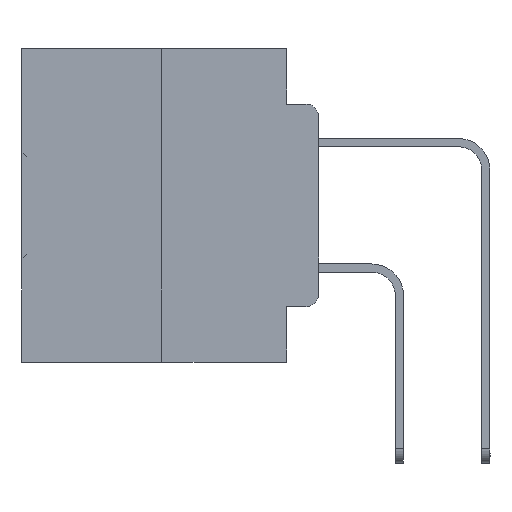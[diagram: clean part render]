
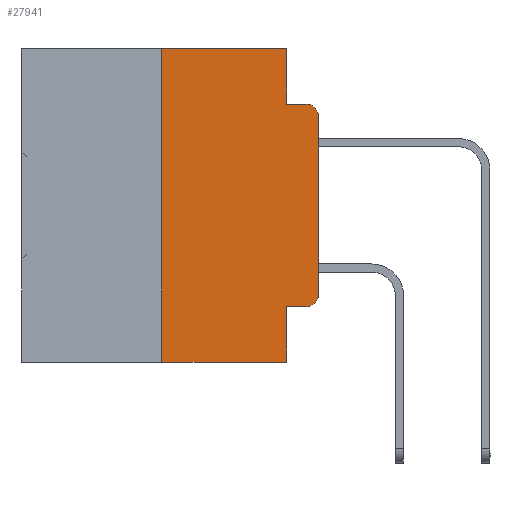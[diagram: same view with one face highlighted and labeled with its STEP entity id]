
A CAD part, left-side view. The second image highlights one B-rep face of the part: STEP entity #27941.
In plain terms, the highlighted planar face has unit normal (-1, 0, 0).
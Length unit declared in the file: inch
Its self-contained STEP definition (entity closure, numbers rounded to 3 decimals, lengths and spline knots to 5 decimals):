
#73 = CARTESIAN_POINT ( 'NONE',  ( 0., 0.051, 0. ) ) ;
#730 = ORIENTED_EDGE ( 'NONE', *, *, #11792, .T. ) ;
#1416 = CARTESIAN_POINT ( 'NONE',  ( 0., 0., -0.3915 ) ) ;
#2061 = DIRECTION ( 'NONE',  ( 0., -1., 0. ) ) ;
#2429 = VERTEX_POINT ( 'NONE', #34743 ) ;
#3399 = DIRECTION ( 'NONE',  ( 0., 0., 1. ) ) ;
#3607 = VECTOR ( 'NONE', #5566, 39.37008 ) ;
#4723 = FACE_OUTER_BOUND ( 'NONE', #28030, .T. ) ;
#5356 = ORIENTED_EDGE ( 'NONE', *, *, #24350, .F. ) ;
#5566 = DIRECTION ( 'NONE',  ( 0., -1., 0. ) ) ;
#7035 = ORIENTED_EDGE ( 'NONE', *, *, #22281, .T. ) ;
#7354 = ORIENTED_EDGE ( 'NONE', *, *, #14879, .F. ) ;
#7501 = LINE ( 'NONE', #73, #13988 ) ;
#7784 = VERTEX_POINT ( 'NONE', #1416 ) ;
#8069 = ORIENTED_EDGE ( 'NONE', *, *, #12528, .F. ) ;
#8354 = AXIS2_PLACEMENT_3D ( 'NONE', #11771, #9117, #33645 ) ;
#8865 = CARTESIAN_POINT ( 'NONE',  ( 0., 0.051, 0. ) ) ;
#8930 = LINE ( 'NONE', #35645, #33581 ) ;
#9117 = DIRECTION ( 'NONE',  ( -1., 0., 0. ) ) ;
#9199 = PLANE ( 'NONE',  #20997 ) ;
#9669 = CARTESIAN_POINT ( 'NONE',  ( 0., 0.25, -0.5 ) ) ;
#10560 = DIRECTION ( 'NONE',  ( 0., 0., -1. ) ) ;
#10842 = CARTESIAN_POINT ( 'NONE',  ( 0., 0.051, -0.4115 ) ) ;
#10954 = DIRECTION ( 'NONE',  ( 0., -1., 0. ) ) ;
#11186 = CARTESIAN_POINT ( 'NONE',  ( 0., 0.473, 0. ) ) ;
#11771 = CARTESIAN_POINT ( 'NONE',  ( 0., 0.02, -0.3915 ) ) ;
#11792 = EDGE_CURVE ( 'NONE', #2429, #7784, #31739, .T. ) ;
#11823 = LINE ( 'NONE', #16718, #3607 ) ;
#12345 = CARTESIAN_POINT ( 'NONE',  ( 0., 0.473, 0. ) ) ;
#12483 = ORIENTED_EDGE ( 'NONE', *, *, #35560, .T. ) ;
#12528 = EDGE_CURVE ( 'NONE', #12726, #15545, #35096, .T. ) ;
#12705 = CIRCLE ( 'NONE', #17532, 0.02 ) ;
#12726 = VERTEX_POINT ( 'NONE', #9669 ) ;
#13062 = VECTOR ( 'NONE', #3399, 39.37008 ) ;
#13065 = VERTEX_POINT ( 'NONE', #8865 ) ;
#13231 = DIRECTION ( 'NONE',  ( -1., 0., 0. ) ) ;
#13613 = CARTESIAN_POINT ( 'NONE',  ( 0., 0.051, -0.4115 ) ) ;
#13663 = CARTESIAN_POINT ( 'NONE',  ( 0., 0.051, -0.0885 ) ) ;
#13988 = VECTOR ( 'NONE', #19879, 39.37008 ) ;
#14879 = EDGE_CURVE ( 'NONE', #13065, #26936, #8930, .T. ) ;
#15179 = VECTOR ( 'NONE', #2061, 39.37008 ) ;
#15545 = VERTEX_POINT ( 'NONE', #25599 ) ;
#15902 = CARTESIAN_POINT ( 'NONE',  ( 0., 0.02, -0.1085 ) ) ;
#16213 = EDGE_CURVE ( 'NONE', #23597, #16334, #12705, .T. ) ;
#16334 = VERTEX_POINT ( 'NONE', #22217 ) ;
#16426 = EDGE_CURVE ( 'NONE', #21245, #32821, #7501, .T. ) ;
#16718 = CARTESIAN_POINT ( 'NONE',  ( 0., 0.473, -0.5 ) ) ;
#17532 = AXIS2_PLACEMENT_3D ( 'NONE', #15902, #13231, #10560 ) ;
#19879 = DIRECTION ( 'NONE',  ( 0., 0., -1. ) ) ;
#20142 = LINE ( 'NONE', #11186, #22800 ) ;
#20997 = AXIS2_PLACEMENT_3D ( 'NONE', #12345, #34086, #23163 ) ;
#21245 = VERTEX_POINT ( 'NONE', #10842 ) ;
#22035 = EDGE_CURVE ( 'NONE', #7784, #23597, #31540, .T. ) ;
#22217 = CARTESIAN_POINT ( 'NONE',  ( 0., 0.02, -0.0885 ) ) ;
#22281 = EDGE_CURVE ( 'NONE', #21245, #2429, #25498, .T. ) ;
#22606 = CARTESIAN_POINT ( 'NONE',  ( 0., 0.051, -0.5 ) ) ;
#22800 = VECTOR ( 'NONE', #10954, 39.37008 ) ;
#22900 = VECTOR ( 'NONE', #30199, 39.37008 ) ;
#23163 = DIRECTION ( 'NONE',  ( 0., 0., -1. ) ) ;
#23359 = CARTESIAN_POINT ( 'NONE',  ( 0., 0., 0. ) ) ;
#23594 = DIRECTION ( 'NONE',  ( 0., 0., 1. ) ) ;
#23597 = VERTEX_POINT ( 'NONE', #35299 ) ;
#24350 = EDGE_CURVE ( 'NONE', #15545, #13065, #20142, .T. ) ;
#24724 = DIRECTION ( 'NONE',  ( 0., 0., -1. ) ) ;
#25498 = LINE ( 'NONE', #13613, #22900 ) ;
#25534 = VECTOR ( 'NONE', #23594, 39.37008 ) ;
#25599 = CARTESIAN_POINT ( 'NONE',  ( 0., 0.25, 0. ) ) ;
#26299 = CARTESIAN_POINT ( 'NONE',  ( 0., 0.051, -0.0885 ) ) ;
#26606 = ORIENTED_EDGE ( 'NONE', *, *, #22035, .T. ) ;
#26936 = VERTEX_POINT ( 'NONE', #26299 ) ;
#27941 = ADVANCED_FACE ( 'NONE', ( #4723 ), #9199, .F. ) ;
#28030 = EDGE_LOOP ( 'NONE', ( #26606, #29717, #30797, #7354, #5356, #8069, #12483, #28763, #7035, #730 ) ) ;
#28159 = LINE ( 'NONE', #13663, #15179 ) ;
#28554 = CARTESIAN_POINT ( 'NONE',  ( 0., 0.25, 0. ) ) ;
#28763 = ORIENTED_EDGE ( 'NONE', *, *, #16426, .F. ) ;
#29717 = ORIENTED_EDGE ( 'NONE', *, *, #16213, .T. ) ;
#30199 = DIRECTION ( 'NONE',  ( 0., -1., 0. ) ) ;
#30797 = ORIENTED_EDGE ( 'NONE', *, *, #34268, .F. ) ;
#31540 = LINE ( 'NONE', #23359, #25534 ) ;
#31739 = CIRCLE ( 'NONE', #8354, 0.02 ) ;
#32821 = VERTEX_POINT ( 'NONE', #22606 ) ;
#33581 = VECTOR ( 'NONE', #24724, 39.37008 ) ;
#33645 = DIRECTION ( 'NONE',  ( 0., 0., -1. ) ) ;
#34086 = DIRECTION ( 'NONE',  ( 1., 0., 0. ) ) ;
#34268 = EDGE_CURVE ( 'NONE', #26936, #16334, #28159, .T. ) ;
#34743 = CARTESIAN_POINT ( 'NONE',  ( 0., 0.02, -0.4115 ) ) ;
#35096 = LINE ( 'NONE', #28554, #13062 ) ;
#35299 = CARTESIAN_POINT ( 'NONE',  ( 0., 0., -0.1085 ) ) ;
#35560 = EDGE_CURVE ( 'NONE', #12726, #32821, #11823, .T. ) ;
#35645 = CARTESIAN_POINT ( 'NONE',  ( 0., 0.051, 0. ) ) ;
